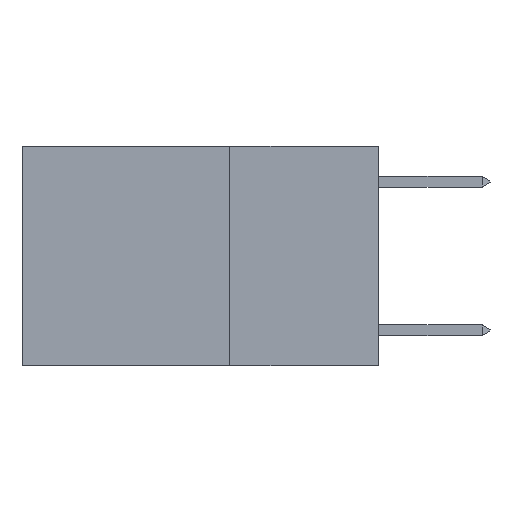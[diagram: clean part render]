
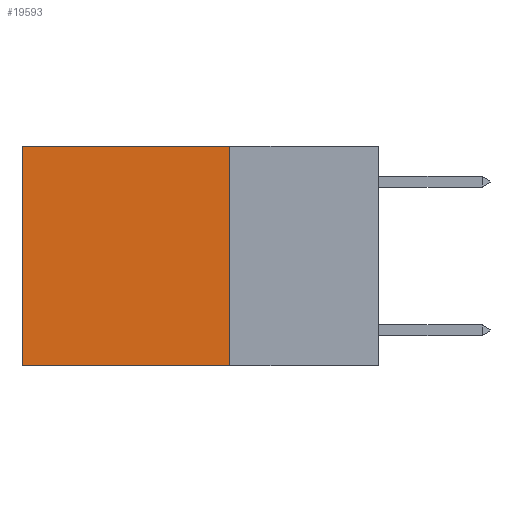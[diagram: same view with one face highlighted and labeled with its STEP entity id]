
A CAD part, left-side view. The second image highlights one B-rep face of the part: STEP entity #19593.
In plain terms, the highlighted planar face has unit normal (-1, 0, 0).
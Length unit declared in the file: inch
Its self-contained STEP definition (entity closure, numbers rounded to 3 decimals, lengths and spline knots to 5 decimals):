
#1347 = DIRECTION ( 'NONE',  ( 0., 0., -1. ) ) ;
#1463 = EDGE_CURVE ( 'NONE', #23849, #14747, #5773, .T. ) ;
#3715 = ORIENTED_EDGE ( 'NONE', *, *, #26163, .F. ) ;
#4135 = CARTESIAN_POINT ( 'NONE',  ( 0.2625, 0.25, 0. ) ) ;
#5506 = VECTOR ( 'NONE', #20327, 39.37008 ) ;
#5773 = LINE ( 'NONE', #23340, #26775 ) ;
#5888 = DIRECTION ( 'NONE',  ( 0., 0., -1. ) ) ;
#8156 = DIRECTION ( 'NONE',  ( 1., 0., 0. ) ) ;
#8179 = CARTESIAN_POINT ( 'NONE',  ( 0.2625, 0.25, 0. ) ) ;
#9665 = EDGE_CURVE ( 'NONE', #24916, #23849, #15860, .T. ) ;
#10098 = CARTESIAN_POINT ( 'NONE',  ( 0.2625, 0.25, 0. ) ) ;
#10406 = DIRECTION ( 'NONE',  ( 0., 0., -1. ) ) ;
#12053 = ORIENTED_EDGE ( 'NONE', *, *, #12307, .F. ) ;
#12307 = EDGE_CURVE ( 'NONE', #19117, #14747, #22520, .T. ) ;
#14747 = VERTEX_POINT ( 'NONE', #14924 ) ;
#14924 = CARTESIAN_POINT ( 'NONE',  ( 0.2625, 0.6, -0.37 ) ) ;
#15091 = PLANE ( 'NONE',  #27890 ) ;
#15806 = EDGE_LOOP ( 'NONE', ( #17673, #12053, #3715, #28395 ) ) ;
#15860 = LINE ( 'NONE', #24640, #5506 ) ;
#17673 = ORIENTED_EDGE ( 'NONE', *, *, #1463, .T. ) ;
#18493 = CARTESIAN_POINT ( 'NONE',  ( 0.2625, 0.25, -0.37 ) ) ;
#19117 = VERTEX_POINT ( 'NONE', #23605 ) ;
#19593 = ADVANCED_FACE ( 'NONE', ( #23430 ), #15091, .F. ) ;
#20327 = DIRECTION ( 'NONE',  ( 0., 1., 0. ) ) ;
#20644 = DIRECTION ( 'NONE',  ( 0., 1., 0. ) ) ;
#22520 = LINE ( 'NONE', #18493, #25370 ) ;
#23340 = CARTESIAN_POINT ( 'NONE',  ( 0.2625, 0.6, 0. ) ) ;
#23430 = FACE_OUTER_BOUND ( 'NONE', #15806, .T. ) ;
#23452 = LINE ( 'NONE', #8179, #25527 ) ;
#23605 = CARTESIAN_POINT ( 'NONE',  ( 0.2625, 0.25, -0.37 ) ) ;
#23849 = VERTEX_POINT ( 'NONE', #24564 ) ;
#24564 = CARTESIAN_POINT ( 'NONE',  ( 0.2625, 0.6, 0. ) ) ;
#24640 = CARTESIAN_POINT ( 'NONE',  ( 0.2625, 0.25, 0. ) ) ;
#24916 = VERTEX_POINT ( 'NONE', #10098 ) ;
#25370 = VECTOR ( 'NONE', #20644, 39.37008 ) ;
#25527 = VECTOR ( 'NONE', #5888, 39.37008 ) ;
#26163 = EDGE_CURVE ( 'NONE', #24916, #19117, #23452, .T. ) ;
#26775 = VECTOR ( 'NONE', #10406, 39.37008 ) ;
#27890 = AXIS2_PLACEMENT_3D ( 'NONE', #4135, #8156, #1347 ) ;
#28395 = ORIENTED_EDGE ( 'NONE', *, *, #9665, .T. ) ;
